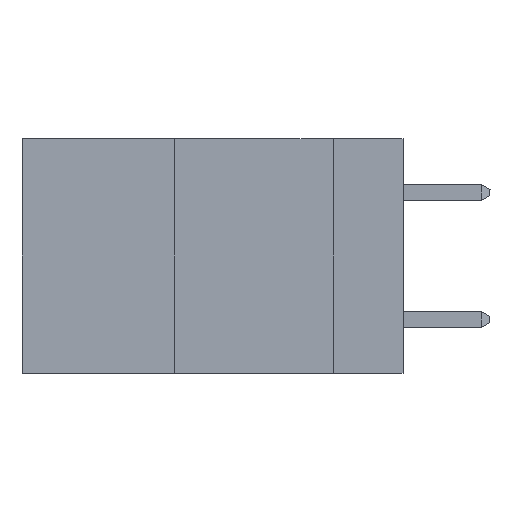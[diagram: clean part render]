
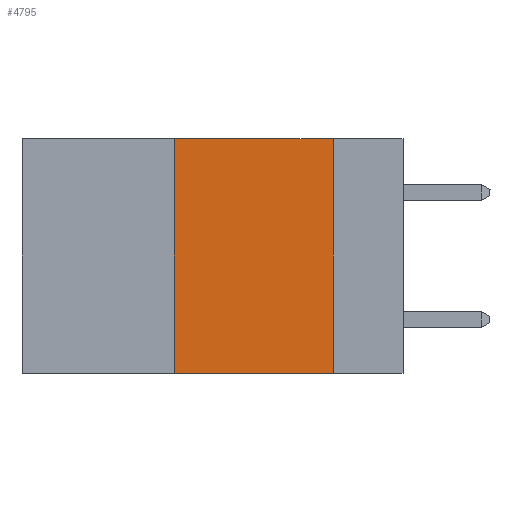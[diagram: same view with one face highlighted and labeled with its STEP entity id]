
A CAD part, left-side view. The second image highlights one B-rep face of the part: STEP entity #4795.
In plain terms, the highlighted planar face has unit normal (-1, 0, 0).
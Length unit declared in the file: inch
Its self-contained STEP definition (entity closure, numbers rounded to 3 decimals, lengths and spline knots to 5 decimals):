
#1828 = EDGE_CURVE ( 'NONE', #14409, #2083, #13087, .T. ) ;
#2083 = VERTEX_POINT ( 'NONE', #13913 ) ;
#2603 = CARTESIAN_POINT ( 'NONE',  ( 0., 0.36, 0. ) ) ;
#2912 = CARTESIAN_POINT ( 'NONE',  ( 0., 0.36, -0.37 ) ) ;
#3091 = CARTESIAN_POINT ( 'NONE',  ( 0., 0.6, 0. ) ) ;
#3119 = ORIENTED_EDGE ( 'NONE', *, *, #1828, .F. ) ;
#3173 = DIRECTION ( 'NONE',  ( 0., 0., -1. ) ) ;
#3883 = CARTESIAN_POINT ( 'NONE',  ( 0., 0.11, 0. ) ) ;
#4280 = ORIENTED_EDGE ( 'NONE', *, *, #4394, .F. ) ;
#4394 = EDGE_CURVE ( 'NONE', #12266, #10226, #11308, .T. ) ;
#4511 = EDGE_LOOP ( 'NONE', ( #3119, #17508, #4280, #19719 ) ) ;
#4795 = ADVANCED_FACE ( 'NONE', ( #18286 ), #10359, .F. ) ;
#5087 = DIRECTION ( 'NONE',  ( 0., -1., 0. ) ) ;
#6186 = EDGE_CURVE ( 'NONE', #10226, #14409, #11231, .T. ) ;
#6408 = VECTOR ( 'NONE', #5087, 39.37008 ) ;
#7871 = VECTOR ( 'NONE', #14949, 39.37008 ) ;
#10226 = VERTEX_POINT ( 'NONE', #2603 ) ;
#10359 = PLANE ( 'NONE',  #11183 ) ;
#10729 = VECTOR ( 'NONE', #21944, 39.37008 ) ;
#11183 = AXIS2_PLACEMENT_3D ( 'NONE', #3091, #14001, #3173 ) ;
#11231 = LINE ( 'NONE', #21156, #6408 ) ;
#11308 = LINE ( 'NONE', #16623, #10729 ) ;
#11412 = CARTESIAN_POINT ( 'NONE',  ( 0., 0.11, 0. ) ) ;
#12266 = VERTEX_POINT ( 'NONE', #2912 ) ;
#13087 = LINE ( 'NONE', #11412, #21987 ) ;
#13190 = CARTESIAN_POINT ( 'NONE',  ( 0., 0.6, -0.37 ) ) ;
#13913 = CARTESIAN_POINT ( 'NONE',  ( 0., 0.11, -0.37 ) ) ;
#14001 = DIRECTION ( 'NONE',  ( 1., 0., 0. ) ) ;
#14409 = VERTEX_POINT ( 'NONE', #3883 ) ;
#14949 = DIRECTION ( 'NONE',  ( 0., -1., 0. ) ) ;
#16623 = CARTESIAN_POINT ( 'NONE',  ( 0., 0.36, 0. ) ) ;
#17445 = LINE ( 'NONE', #13190, #7871 ) ;
#17508 = ORIENTED_EDGE ( 'NONE', *, *, #6186, .F. ) ;
#18286 = FACE_OUTER_BOUND ( 'NONE', #4511, .T. ) ;
#19719 = ORIENTED_EDGE ( 'NONE', *, *, #20702, .T. ) ;
#20702 = EDGE_CURVE ( 'NONE', #12266, #2083, #17445, .T. ) ;
#21156 = CARTESIAN_POINT ( 'NONE',  ( 0., 0.6, 0. ) ) ;
#21944 = DIRECTION ( 'NONE',  ( 0., 0., 1. ) ) ;
#21987 = VECTOR ( 'NONE', #22072, 39.37008 ) ;
#22072 = DIRECTION ( 'NONE',  ( 0., 0., -1. ) ) ;
